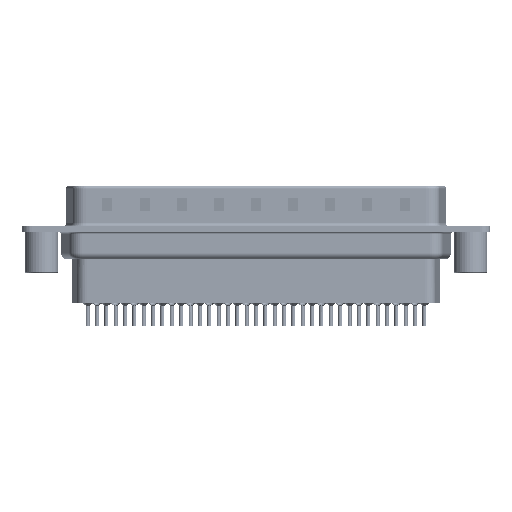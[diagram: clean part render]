
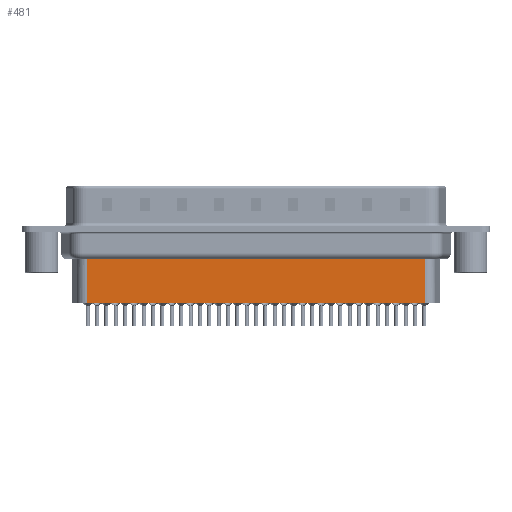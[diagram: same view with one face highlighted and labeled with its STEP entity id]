
A CAD part, front view. The second image highlights one B-rep face of the part: STEP entity #481.
In plain terms, the highlighted planar face has unit normal (0, -1, 0).
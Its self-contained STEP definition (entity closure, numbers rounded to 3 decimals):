
#481 = ADVANCED_FACE ( 'NONE', ( #8993 ), #15709, .T. ) ;
#943 = VECTOR ( 'NONE', #4863, 1000. ) ;
#1636 = VERTEX_POINT ( 'NONE', #26066 ) ;
#2414 = CARTESIAN_POINT ( 'NONE',  ( 6.459, -3.5, -4.097 ) ) ;
#3997 = EDGE_CURVE ( 'NONE', #29114, #1636, #15203, .T. ) ;
#4196 = CARTESIAN_POINT ( 'NONE',  ( 56.794, -3.5, -3.1 ) ) ;
#4287 = CARTESIAN_POINT ( 'NONE',  ( 6.706, -3.5, -3.1 ) ) ;
#4708 = DIRECTION ( 'NONE',  ( -1., 0., 0. ) ) ;
#4863 = DIRECTION ( 'NONE',  ( -1., 0., 0. ) ) ;
#5397 = CARTESIAN_POINT ( 'NONE',  ( 56.794, -3.5, -10.95 ) ) ;
#5928 = ORIENTED_EDGE ( 'NONE', *, *, #15513, .F. ) ;
#7110 = ORIENTED_EDGE ( 'NONE', *, *, #15546, .T. ) ;
#8710 = CARTESIAN_POINT ( 'NONE',  ( 56.794, -3.5, -4.097 ) ) ;
#8803 = LINE ( 'NONE', #25399, #943 ) ;
#8993 = FACE_OUTER_BOUND ( 'NONE', #29276, .T. ) ;
#9848 = VECTOR ( 'NONE', #20219, 1000. ) ;
#10825 = ORIENTED_EDGE ( 'NONE', *, *, #3997, .T. ) ;
#12599 = CARTESIAN_POINT ( 'NONE',  ( 6.706, -3.5, -3.1 ) ) ;
#13107 = VECTOR ( 'NONE', #4708, 1000. ) ;
#14617 = ORIENTED_EDGE ( 'NONE', *, *, #29703, .F. ) ;
#15203 = LINE ( 'NONE', #12599, #9848 ) ;
#15513 = EDGE_CURVE ( 'NONE', #29839, #1636, #8803, .T. ) ;
#15546 = EDGE_CURVE ( 'NONE', #28937, #29114, #18100, .T. ) ;
#15709 = PLANE ( 'NONE',  #25233 ) ;
#18042 = LINE ( 'NONE', #4196, #22905 ) ;
#18100 = LINE ( 'NONE', #2414, #13107 ) ;
#18282 = DIRECTION ( 'NONE',  ( 0., -1., 0. ) ) ;
#20219 = DIRECTION ( 'NONE',  ( 0., 0., -1. ) ) ;
#20947 = DIRECTION ( 'NONE',  ( 0., 0., -1. ) ) ;
#22905 = VECTOR ( 'NONE', #20947, 1000. ) ;
#24980 = DIRECTION ( 'NONE',  ( 1., 0., 0. ) ) ;
#25233 = AXIS2_PLACEMENT_3D ( 'NONE', #4287, #18282, #24980 ) ;
#25399 = CARTESIAN_POINT ( 'NONE',  ( 6.706, -3.5, -10.95 ) ) ;
#26066 = CARTESIAN_POINT ( 'NONE',  ( 6.706, -3.5, -10.95 ) ) ;
#28937 = VERTEX_POINT ( 'NONE', #8710 ) ;
#29114 = VERTEX_POINT ( 'NONE', #29325 ) ;
#29276 = EDGE_LOOP ( 'NONE', ( #14617, #7110, #10825, #5928 ) ) ;
#29325 = CARTESIAN_POINT ( 'NONE',  ( 6.706, -3.5, -4.097 ) ) ;
#29703 = EDGE_CURVE ( 'NONE', #28937, #29839, #18042, .T. ) ;
#29839 = VERTEX_POINT ( 'NONE', #5397 ) ;
